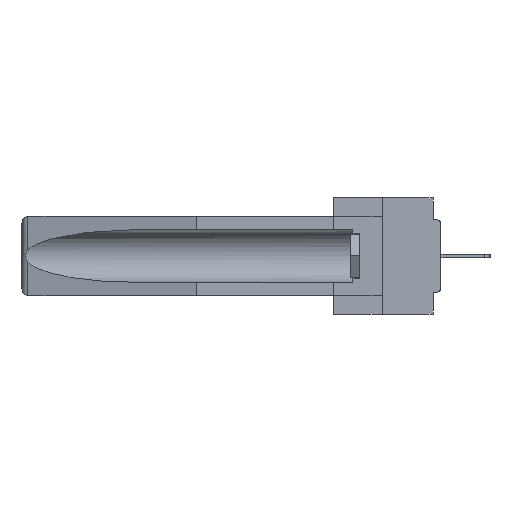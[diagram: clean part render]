
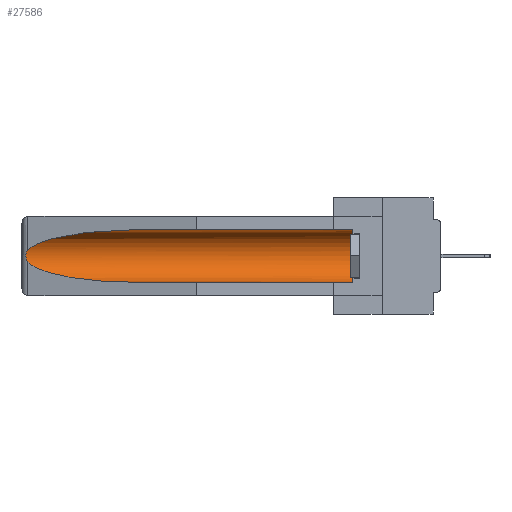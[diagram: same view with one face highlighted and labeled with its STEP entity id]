
A CAD part, left-side view. The second image highlights one B-rep face of the part: STEP entity #27586.
In plain terms, the highlighted cylindrical face has radius 2.857 mm (diameter 5.715 mm), a partial arc.
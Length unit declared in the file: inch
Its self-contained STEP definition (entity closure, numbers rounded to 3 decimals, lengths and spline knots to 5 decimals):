
#72 = CARTESIAN_POINT ( 'NONE',  ( 0.2675, 1.53308, -0.17534 ) ) ;
#250 = CARTESIAN_POINT ( 'NONE',  ( 0.2675, 1.53308, -0.16763 ) ) ;
#417 = CARTESIAN_POINT ( 'NONE',  ( 0.26537, 1.52718, -0.14972 ) ) ;
#508 = CARTESIAN_POINT ( 'NONE',  ( 0.155, 0.126, -0.1715 ) ) ;
#1305 = CARTESIAN_POINT ( 'NONE',  ( 0.155, 1.07973, -0.284 ) ) ;
#1566 = DIRECTION ( 'NONE',  ( 0., 1., 0. ) ) ;
#2156 = CARTESIAN_POINT ( 'NONE',  ( 0.26537, 1.52718, -0.19328 ) ) ;
#2768 = CARTESIAN_POINT ( 'NONE',  ( 0.26537, 1.52718, -0.14972 ) ) ;
#3937 = ORIENTED_EDGE ( 'NONE', *, *, #11374, .T. ) ;
#4853 = EDGE_CURVE ( 'NONE', #31283, #13277, #13716, .T. ) ;
#7062 = VECTOR ( 'NONE', #1566, 39.37008 ) ;
#8369 = CARTESIAN_POINT ( 'NONE',  ( 0.155, 0.126, -0.284 ) ) ;
#9526 = B_SPLINE_CURVE_WITH_KNOTS ( 'NONE', 3,
 ( #2768, #31324, #16965, #16780, #250, #72, #17148, #14230, #11314, #16604 ),
 .UNSPECIFIED., .F., .F.,
 ( 4, 2, 2, 2, 4 ),
 ( 0., 0.00029, 0.00058, 0.00087, 0.00117 ),
 .UNSPECIFIED. ) ;
#9754 = CARTESIAN_POINT ( 'NONE',  ( 0.155, -0.30754, -0.059 ) ) ;
#11033 = CARTESIAN_POINT ( 'NONE',  ( 0.25451, 1.48313, -0.24835 ) ) ;
#11314 = CARTESIAN_POINT ( 'NONE',  ( 0.26597, 1.5296, -0.19026 ) ) ;
#11374 = EDGE_CURVE ( 'NONE', #30742, #13486, #27197, .T. ) ;
#11764 = DIRECTION ( 'NONE',  ( 0., -1., 0. ) ) ;
#11825 = ORIENTED_EDGE ( 'NONE', *, *, #4853, .F. ) ;
#12759 = EDGE_CURVE ( 'NONE', #23659, #13277, #16626, .T. ) ;
#12859 = ORIENTED_EDGE ( 'NONE', *, *, #24085, .T. ) ;
#13277 = VERTEX_POINT ( 'NONE', #1305 ) ;
#13406 = ORIENTED_EDGE ( 'NONE', *, *, #31661, .T. ) ;
#13486 = VERTEX_POINT ( 'NONE', #21664 ) ;
#13607 = CARTESIAN_POINT ( 'NONE',  ( 0.26537, 1.52718, -0.14972 ) ) ;
#13716 = LINE ( 'NONE', #18648, #24701 ) ;
#14230 = CARTESIAN_POINT ( 'NONE',  ( 0.26655, 1.53094, -0.18657 ) ) ;
#14513 = AXIS2_PLACEMENT_3D ( 'NONE', #508, #11764, #19968 ) ;
#16604 = CARTESIAN_POINT ( 'NONE',  ( 0.26537, 1.52718, -0.19328 ) ) ;
#16626 =( BOUNDED_CURVE ( )  B_SPLINE_CURVE ( 3, ( #27244, #11033, #30159, #22138 ),
 .UNSPECIFIED., .F., .F. ) 
 B_SPLINE_CURVE_WITH_KNOTS ( ( 4, 4 ),
 ( 0.1948, 1.5708 ),
 .UNSPECIFIED. ) 
 CURVE ( )  GEOMETRIC_REPRESENTATION_ITEM ( )  RATIONAL_B_SPLINE_CURVE ( ( 1., 0.848, 0.848, 1. ) ) 
 REPRESENTATION_ITEM ( '' )  );
#16780 = CARTESIAN_POINT ( 'NONE',  ( 0.2673, 1.5327, -0.16383 ) ) ;
#16965 = CARTESIAN_POINT ( 'NONE',  ( 0.26654, 1.53092, -0.15636 ) ) ;
#17148 = CARTESIAN_POINT ( 'NONE',  ( 0.2673, 1.53269, -0.17917 ) ) ;
#18648 = CARTESIAN_POINT ( 'NONE',  ( 0.155, -0.30754, -0.284 ) ) ;
#18800 = CARTESIAN_POINT ( 'NONE',  ( 0.155, 0.126, -0.059 ) ) ;
#19249 = CARTESIAN_POINT ( 'NONE',  ( 0.25451, 1.48313, -0.09465 ) ) ;
#19968 = DIRECTION ( 'NONE',  ( 0., 0., 1. ) ) ;
#20583 = DIRECTION ( 'NONE',  ( 0., 0., 1. ) ) ;
#20797 = EDGE_LOOP ( 'NONE', ( #13406, #12859, #21750, #11825, #33672, #3937 ) ) ;
#20936 = CARTESIAN_POINT ( 'NONE',  ( 0.155, -0.30754, -0.1715 ) ) ;
#21664 = CARTESIAN_POINT ( 'NONE',  ( 0.155, 1.07973, -0.059 ) ) ;
#21750 = ORIENTED_EDGE ( 'NONE', *, *, #12759, .T. ) ;
#21803 = CARTESIAN_POINT ( 'NONE',  ( 0.21114, 1.30732, -0.059 ) ) ;
#22138 = CARTESIAN_POINT ( 'NONE',  ( 0.155, 1.07973, -0.284 ) ) ;
#22442 = FACE_OUTER_BOUND ( 'NONE', #20797, .T. ) ;
#22923 = VERTEX_POINT ( 'NONE', #417 ) ;
#23659 = VERTEX_POINT ( 'NONE', #2156 ) ;
#24085 = EDGE_CURVE ( 'NONE', #22923, #23659, #9526, .T. ) ;
#24701 = VECTOR ( 'NONE', #33193, 39.37008 ) ;
#27197 = LINE ( 'NONE', #9754, #7062 ) ;
#27244 = CARTESIAN_POINT ( 'NONE',  ( 0.26537, 1.52718, -0.19328 ) ) ;
#27586 = ADVANCED_FACE ( 'NONE', ( #22442 ), #31658, .F. ) ;
#27888 = AXIS2_PLACEMENT_3D ( 'NONE', #20936, #34768, #20583 ) ;
#30007 = EDGE_CURVE ( 'NONE', #31283, #30742, #30213, .T. ) ;
#30159 = CARTESIAN_POINT ( 'NONE',  ( 0.21114, 1.30732, -0.284 ) ) ;
#30213 = CIRCLE ( 'NONE', #14513, 0.1125 ) ;
#30345 =( BOUNDED_CURVE ( )  B_SPLINE_CURVE ( 3, ( #32902, #21803, #19249, #13607 ),
 .UNSPECIFIED., .F., .F. ) 
 B_SPLINE_CURVE_WITH_KNOTS ( ( 4, 4 ),
 ( 4.71239, 6.08839 ),
 .UNSPECIFIED. ) 
 CURVE ( )  GEOMETRIC_REPRESENTATION_ITEM ( )  RATIONAL_B_SPLINE_CURVE ( ( 1., 0.848, 0.848, 1. ) ) 
 REPRESENTATION_ITEM ( '' )  );
#30742 = VERTEX_POINT ( 'NONE', #18800 ) ;
#31283 = VERTEX_POINT ( 'NONE', #8369 ) ;
#31324 = CARTESIAN_POINT ( 'NONE',  ( 0.26597, 1.52961, -0.15275 ) ) ;
#31658 = CYLINDRICAL_SURFACE ( 'NONE', #27888, 0.1125 ) ;
#31661 = EDGE_CURVE ( 'NONE', #13486, #22923, #30345, .T. ) ;
#32902 = CARTESIAN_POINT ( 'NONE',  ( 0.155, 1.07973, -0.059 ) ) ;
#33193 = DIRECTION ( 'NONE',  ( 0., 1., 0. ) ) ;
#33672 = ORIENTED_EDGE ( 'NONE', *, *, #30007, .T. ) ;
#34768 = DIRECTION ( 'NONE',  ( 0., 1., 0. ) ) ;
